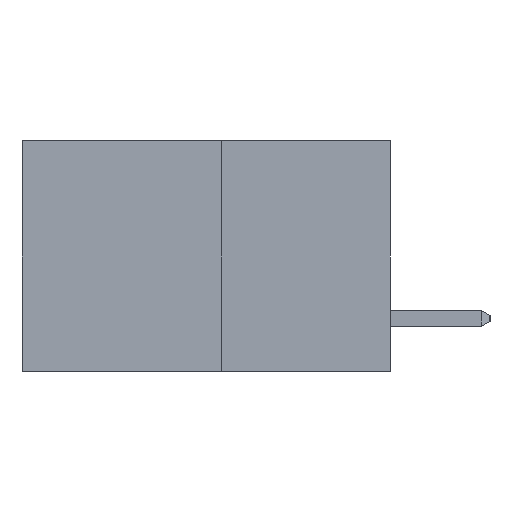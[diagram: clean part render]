
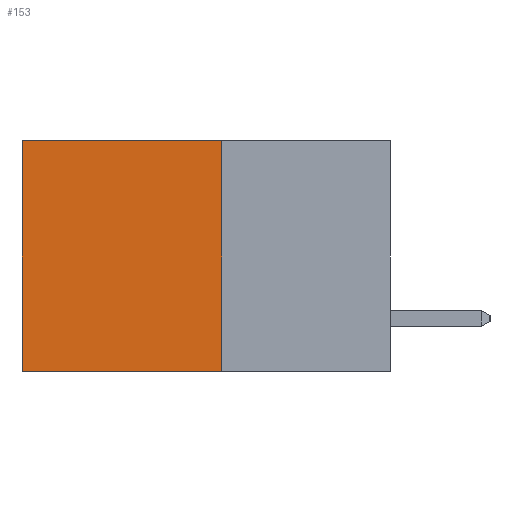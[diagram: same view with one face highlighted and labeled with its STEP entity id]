
A CAD part, left-side view. The second image highlights one B-rep face of the part: STEP entity #153.
In plain terms, the highlighted planar face has unit normal (-1, 0, 0).
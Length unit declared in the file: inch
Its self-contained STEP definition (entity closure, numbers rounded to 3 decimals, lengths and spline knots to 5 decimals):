
#100 = VERTEX_POINT ( 'NONE', #11702 ) ;
#153 = ADVANCED_FACE ( 'NONE', ( #10451 ), #14680, .F. ) ;
#201 = VECTOR ( 'NONE', #14088, 39.37008 ) ;
#528 = CARTESIAN_POINT ( 'NONE',  ( 0.277, 0.59, -0.37 ) ) ;
#760 = EDGE_CURVE ( 'NONE', #100, #6746, #10593, .T. ) ;
#828 = ORIENTED_EDGE ( 'NONE', *, *, #12427, .T. ) ;
#890 = VECTOR ( 'NONE', #10200, 39.37008 ) ;
#1429 = DIRECTION ( 'NONE',  ( 0., 1., 0. ) ) ;
#1786 = CARTESIAN_POINT ( 'NONE',  ( 0.277, 0.59, 0. ) ) ;
#3377 = EDGE_CURVE ( 'NONE', #6746, #9617, #5680, .T. ) ;
#4115 = LINE ( 'NONE', #4365, #9990 ) ;
#4332 = DIRECTION ( 'NONE',  ( 0., 0., -1. ) ) ;
#4365 = CARTESIAN_POINT ( 'NONE',  ( 0.277, 0.59, -0.37 ) ) ;
#4657 = ORIENTED_EDGE ( 'NONE', *, *, #3377, .F. ) ;
#5383 = ORIENTED_EDGE ( 'NONE', *, *, #12004, .T. ) ;
#5680 = LINE ( 'NONE', #13874, #8797 ) ;
#6495 = LINE ( 'NONE', #12962, #201 ) ;
#6699 = DIRECTION ( 'NONE',  ( 0., 0., -1. ) ) ;
#6746 = VERTEX_POINT ( 'NONE', #10301 ) ;
#7824 = DIRECTION ( 'NONE',  ( 1., 0., 0. ) ) ;
#8797 = VECTOR ( 'NONE', #1429, 39.37008 ) ;
#9275 = CARTESIAN_POINT ( 'NONE',  ( 0.277, 0.27, -0.37 ) ) ;
#9617 = VERTEX_POINT ( 'NONE', #528 ) ;
#9958 = AXIS2_PLACEMENT_3D ( 'NONE', #9275, #7824, #4332 ) ;
#9990 = VECTOR ( 'NONE', #6699, 39.37008 ) ;
#10162 = CARTESIAN_POINT ( 'NONE',  ( 0.277, 0.27, -0.37 ) ) ;
#10200 = DIRECTION ( 'NONE',  ( 0., 0., -1. ) ) ;
#10301 = CARTESIAN_POINT ( 'NONE',  ( 0.277, 0.27, -0.37 ) ) ;
#10451 = FACE_OUTER_BOUND ( 'NONE', #14804, .T. ) ;
#10593 = LINE ( 'NONE', #10162, #890 ) ;
#11258 = ORIENTED_EDGE ( 'NONE', *, *, #760, .F. ) ;
#11702 = CARTESIAN_POINT ( 'NONE',  ( 0.277, 0.27, 0. ) ) ;
#12004 = EDGE_CURVE ( 'NONE', #100, #13101, #6495, .T. ) ;
#12427 = EDGE_CURVE ( 'NONE', #13101, #9617, #4115, .T. ) ;
#12962 = CARTESIAN_POINT ( 'NONE',  ( 0.277, 0.27, 0. ) ) ;
#13101 = VERTEX_POINT ( 'NONE', #1786 ) ;
#13874 = CARTESIAN_POINT ( 'NONE',  ( 0.277, 0.27, -0.37 ) ) ;
#14088 = DIRECTION ( 'NONE',  ( 0., 1., 0. ) ) ;
#14680 = PLANE ( 'NONE',  #9958 ) ;
#14804 = EDGE_LOOP ( 'NONE', ( #828, #4657, #11258, #5383 ) ) ;
